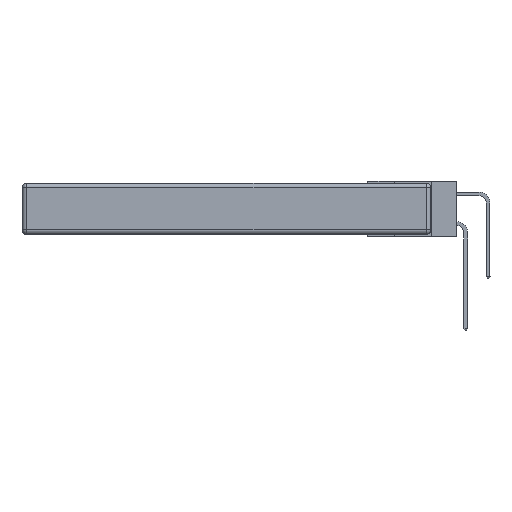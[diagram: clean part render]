
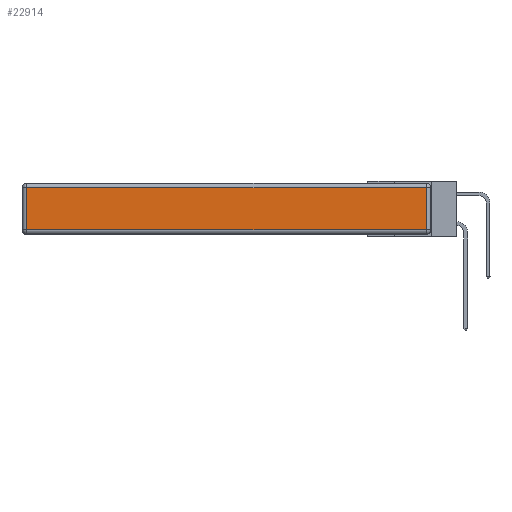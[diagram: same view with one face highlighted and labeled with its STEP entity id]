
A CAD part, left-side view. The second image highlights one B-rep face of the part: STEP entity #22914.
In plain terms, the highlighted planar face has unit normal (-1, 0, 0).
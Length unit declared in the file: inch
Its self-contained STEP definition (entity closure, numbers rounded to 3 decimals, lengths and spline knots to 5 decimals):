
#254 = ORIENTED_EDGE ( 'NONE', *, *, #21910, .T. ) ;
#1779 = DIRECTION ( 'NONE',  ( 0., 0., 1. ) ) ;
#1903 = CARTESIAN_POINT ( 'NONE',  ( 0., 0.03, -0.343 ) ) ;
#2013 = CARTESIAN_POINT ( 'NONE',  ( 0., 0., -0.343 ) ) ;
#4562 = VECTOR ( 'NONE', #11814, 39.37008 ) ;
#4583 = CARTESIAN_POINT ( 'NONE',  ( 0., 2.72, -0.03 ) ) ;
#5541 = VECTOR ( 'NONE', #1779, 39.37008 ) ;
#5965 = ORIENTED_EDGE ( 'NONE', *, *, #10166, .T. ) ;
#6557 = LINE ( 'NONE', #27991, #19287 ) ;
#10166 = EDGE_CURVE ( 'NONE', #14427, #18273, #6557, .T. ) ;
#10556 = DIRECTION ( 'NONE',  ( 0., -1., 0. ) ) ;
#10757 = EDGE_CURVE ( 'NONE', #26612, #25472, #11585, .T. ) ;
#11585 = LINE ( 'NONE', #13431, #31715 ) ;
#11814 = DIRECTION ( 'NONE',  ( 0., 0., -1. ) ) ;
#12657 = ORIENTED_EDGE ( 'NONE', *, *, #34331, .T. ) ;
#13431 = CARTESIAN_POINT ( 'NONE',  ( 0., 0., -0.313 ) ) ;
#14427 = VERTEX_POINT ( 'NONE', #30421 ) ;
#16815 = FACE_OUTER_BOUND ( 'NONE', #30413, .T. ) ;
#17603 = ORIENTED_EDGE ( 'NONE', *, *, #10757, .T. ) ;
#18273 = VERTEX_POINT ( 'NONE', #4583 ) ;
#19287 = VECTOR ( 'NONE', #28107, 39.37008 ) ;
#19998 = LINE ( 'NONE', #1903, #5541 ) ;
#20499 = CARTESIAN_POINT ( 'NONE',  ( 0., 2.72, -0.313 ) ) ;
#21074 = DIRECTION ( 'NONE',  ( -1., 0., 0. ) ) ;
#21910 = EDGE_CURVE ( 'NONE', #18273, #26612, #30169, .T. ) ;
#22914 = ADVANCED_FACE ( 'NONE', ( #16815 ), #29111, .T. ) ;
#25160 = CARTESIAN_POINT ( 'NONE',  ( 0., 0.03, -0.313 ) ) ;
#25472 = VERTEX_POINT ( 'NONE', #25160 ) ;
#26612 = VERTEX_POINT ( 'NONE', #20499 ) ;
#27991 = CARTESIAN_POINT ( 'NONE',  ( 0., 2.75, -0.03 ) ) ;
#28107 = DIRECTION ( 'NONE',  ( 0., 1., 0. ) ) ;
#29111 = PLANE ( 'NONE',  #31337 ) ;
#30169 = LINE ( 'NONE', #30303, #4562 ) ;
#30303 = CARTESIAN_POINT ( 'NONE',  ( 0., 2.72, -0.343 ) ) ;
#30413 = EDGE_LOOP ( 'NONE', ( #17603, #12657, #5965, #254 ) ) ;
#30421 = CARTESIAN_POINT ( 'NONE',  ( 0., 0.03, -0.03 ) ) ;
#31337 = AXIS2_PLACEMENT_3D ( 'NONE', #2013, #21074, #31849 ) ;
#31715 = VECTOR ( 'NONE', #10556, 39.37008 ) ;
#31849 = DIRECTION ( 'NONE',  ( 0., 0., 1. ) ) ;
#34331 = EDGE_CURVE ( 'NONE', #25472, #14427, #19998, .T. ) ;
